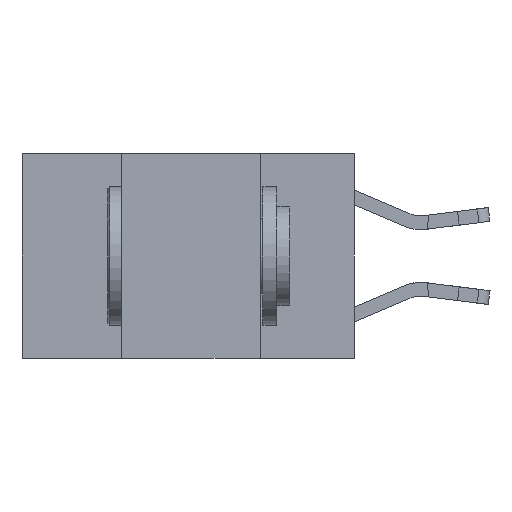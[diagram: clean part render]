
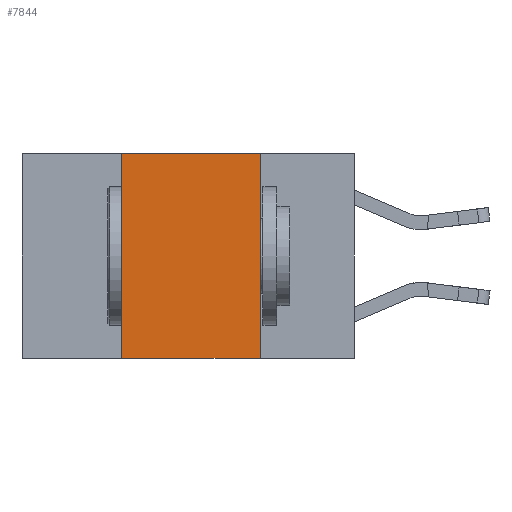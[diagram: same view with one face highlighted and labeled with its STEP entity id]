
A CAD part, left-side view. The second image highlights one B-rep face of the part: STEP entity #7844.
In plain terms, the highlighted planar face has unit normal (-1, 0, 0).
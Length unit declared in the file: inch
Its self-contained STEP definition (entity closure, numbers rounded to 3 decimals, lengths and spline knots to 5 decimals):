
#971 = EDGE_CURVE ( 'NONE', #2207, #9979, #6306, .T. ) ;
#1386 = DIRECTION ( 'NONE',  ( 0., -1., 0. ) ) ;
#1503 = CARTESIAN_POINT ( 'NONE',  ( 0., 0.17, 0. ) ) ;
#2207 = VERTEX_POINT ( 'NONE', #5562 ) ;
#2349 = CARTESIAN_POINT ( 'NONE',  ( 0., 0.42, 0. ) ) ;
#4775 = VECTOR ( 'NONE', #15629, 39.37008 ) ;
#5532 = LINE ( 'NONE', #11238, #16856 ) ;
#5540 = EDGE_CURVE ( 'NONE', #8398, #2207, #8457, .T. ) ;
#5562 = CARTESIAN_POINT ( 'NONE',  ( 0., 0.17, 0. ) ) ;
#6306 = LINE ( 'NONE', #1503, #4775 ) ;
#6992 = VECTOR ( 'NONE', #13875, 39.37008 ) ;
#7056 = EDGE_LOOP ( 'NONE', ( #10574, #7886, #11716, #17187 ) ) ;
#7385 = FACE_OUTER_BOUND ( 'NONE', #7056, .T. ) ;
#7746 = DIRECTION ( 'NONE',  ( 1., 0., 0. ) ) ;
#7844 = ADVANCED_FACE ( 'NONE', ( #7385 ), #11965, .F. ) ;
#7886 = ORIENTED_EDGE ( 'NONE', *, *, #5540, .F. ) ;
#8398 = VERTEX_POINT ( 'NONE', #2349 ) ;
#8457 = LINE ( 'NONE', #14485, #16324 ) ;
#8537 = DIRECTION ( 'NONE',  ( 0., 0., 1. ) ) ;
#8993 = CARTESIAN_POINT ( 'NONE',  ( 0., 0.42, -0.37 ) ) ;
#9979 = VERTEX_POINT ( 'NONE', #17385 ) ;
#10387 = CARTESIAN_POINT ( 'NONE',  ( 0., 0.6, 0. ) ) ;
#10574 = ORIENTED_EDGE ( 'NONE', *, *, #971, .F. ) ;
#10948 = CARTESIAN_POINT ( 'NONE',  ( 0., 0.6, -0.37 ) ) ;
#11238 = CARTESIAN_POINT ( 'NONE',  ( 0., 0.42, 0. ) ) ;
#11242 = EDGE_CURVE ( 'NONE', #15536, #8398, #5532, .T. ) ;
#11716 = ORIENTED_EDGE ( 'NONE', *, *, #11242, .F. ) ;
#11965 = PLANE ( 'NONE',  #14655 ) ;
#13296 = DIRECTION ( 'NONE',  ( 0., 0., -1. ) ) ;
#13875 = DIRECTION ( 'NONE',  ( 0., -1., 0. ) ) ;
#14485 = CARTESIAN_POINT ( 'NONE',  ( 0., 0.6, 0. ) ) ;
#14655 = AXIS2_PLACEMENT_3D ( 'NONE', #10387, #7746, #13296 ) ;
#15536 = VERTEX_POINT ( 'NONE', #8993 ) ;
#15602 = EDGE_CURVE ( 'NONE', #15536, #9979, #16719, .T. ) ;
#15629 = DIRECTION ( 'NONE',  ( 0., 0., -1. ) ) ;
#16324 = VECTOR ( 'NONE', #1386, 39.37008 ) ;
#16719 = LINE ( 'NONE', #10948, #6992 ) ;
#16856 = VECTOR ( 'NONE', #8537, 39.37008 ) ;
#17187 = ORIENTED_EDGE ( 'NONE', *, *, #15602, .T. ) ;
#17385 = CARTESIAN_POINT ( 'NONE',  ( 0., 0.17, -0.37 ) ) ;
